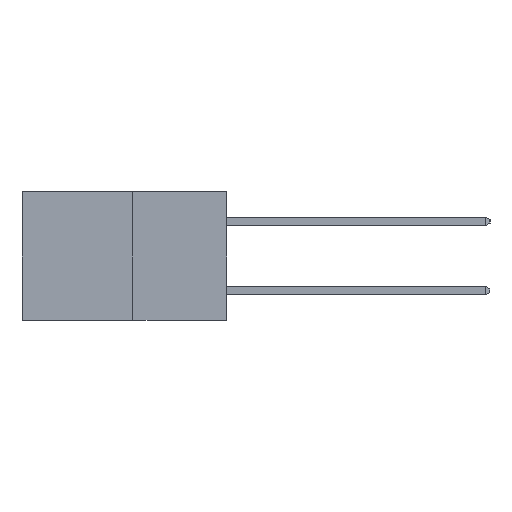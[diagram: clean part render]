
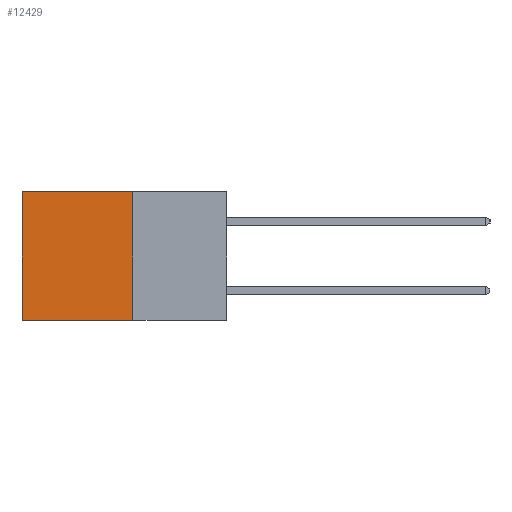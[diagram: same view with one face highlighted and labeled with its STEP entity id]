
A CAD part, left-side view. The second image highlights one B-rep face of the part: STEP entity #12429.
In plain terms, the highlighted planar face has unit normal (-1, 0, 0).
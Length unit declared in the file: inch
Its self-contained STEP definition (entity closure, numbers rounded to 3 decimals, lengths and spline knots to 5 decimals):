
#1657 = CARTESIAN_POINT ( 'NONE',  ( 0.277, 0.27, -0.37 ) ) ;
#2298 = CARTESIAN_POINT ( 'NONE',  ( 0.277, 0.27, 0. ) ) ;
#2391 = EDGE_CURVE ( 'NONE', #8145, #10332, #16459, .T. ) ;
#2506 = FACE_OUTER_BOUND ( 'NONE', #2851, .T. ) ;
#2851 = EDGE_LOOP ( 'NONE', ( #8948, #18727, #17953, #19699 ) ) ;
#2867 = DIRECTION ( 'NONE',  ( 0., 0., -1. ) ) ;
#3954 = VECTOR ( 'NONE', #13789, 39.37008 ) ;
#4371 = LINE ( 'NONE', #10521, #21261 ) ;
#4456 = LINE ( 'NONE', #2298, #3954 ) ;
#5370 = CARTESIAN_POINT ( 'NONE',  ( 0.277, 0.59, -0.37 ) ) ;
#6021 = CARTESIAN_POINT ( 'NONE',  ( 0.277, 0.27, -0.37 ) ) ;
#6804 = LINE ( 'NONE', #16013, #19412 ) ;
#7310 = CARTESIAN_POINT ( 'NONE',  ( 0.277, 0.59, -0.37 ) ) ;
#7639 = CARTESIAN_POINT ( 'NONE',  ( 0.277, 0.59, 0. ) ) ;
#7651 = DIRECTION ( 'NONE',  ( 1., 0., 0. ) ) ;
#8145 = VERTEX_POINT ( 'NONE', #7639 ) ;
#8185 = VECTOR ( 'NONE', #11174, 39.37008 ) ;
#8948 = ORIENTED_EDGE ( 'NONE', *, *, #2391, .T. ) ;
#9569 = EDGE_CURVE ( 'NONE', #13204, #11320, #6804, .T. ) ;
#10332 = VERTEX_POINT ( 'NONE', #7310 ) ;
#10521 = CARTESIAN_POINT ( 'NONE',  ( 0.277, 0.27, -0.37 ) ) ;
#11174 = DIRECTION ( 'NONE',  ( 0., 0., -1. ) ) ;
#11320 = VERTEX_POINT ( 'NONE', #1657 ) ;
#12429 = ADVANCED_FACE ( 'NONE', ( #2506 ), #15866, .F. ) ;
#13204 = VERTEX_POINT ( 'NONE', #19218 ) ;
#13789 = DIRECTION ( 'NONE',  ( 0., 1., 0. ) ) ;
#14172 = AXIS2_PLACEMENT_3D ( 'NONE', #6021, #7651, #19176 ) ;
#15109 = EDGE_CURVE ( 'NONE', #13204, #8145, #4456, .T. ) ;
#15866 = PLANE ( 'NONE',  #14172 ) ;
#16013 = CARTESIAN_POINT ( 'NONE',  ( 0.277, 0.27, -0.37 ) ) ;
#16459 = LINE ( 'NONE', #5370, #8185 ) ;
#17953 = ORIENTED_EDGE ( 'NONE', *, *, #9569, .F. ) ;
#18727 = ORIENTED_EDGE ( 'NONE', *, *, #20277, .F. ) ;
#19176 = DIRECTION ( 'NONE',  ( 0., 0., -1. ) ) ;
#19218 = CARTESIAN_POINT ( 'NONE',  ( 0.277, 0.27, 0. ) ) ;
#19412 = VECTOR ( 'NONE', #2867, 39.37008 ) ;
#19699 = ORIENTED_EDGE ( 'NONE', *, *, #15109, .T. ) ;
#20277 = EDGE_CURVE ( 'NONE', #11320, #10332, #4371, .T. ) ;
#20370 = DIRECTION ( 'NONE',  ( 0., 1., 0. ) ) ;
#21261 = VECTOR ( 'NONE', #20370, 39.37008 ) ;
